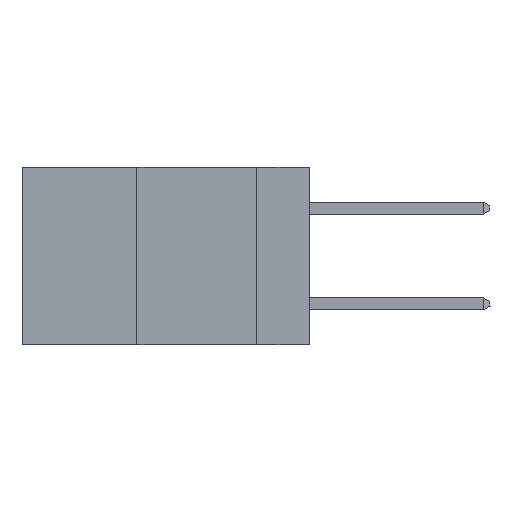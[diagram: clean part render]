
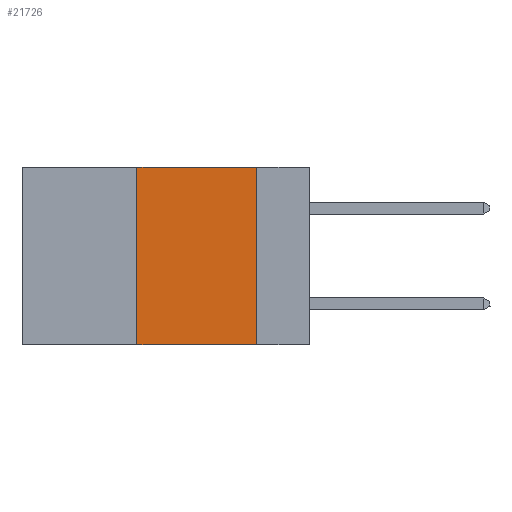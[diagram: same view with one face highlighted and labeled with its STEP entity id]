
A CAD part, left-side view. The second image highlights one B-rep face of the part: STEP entity #21726.
In plain terms, the highlighted planar face has unit normal (-1, 0, 0).
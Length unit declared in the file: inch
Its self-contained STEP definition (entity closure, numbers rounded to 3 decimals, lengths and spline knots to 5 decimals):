
#480 = DIRECTION ( 'NONE',  ( 0., -1., 0. ) ) ;
#1325 = LINE ( 'NONE', #21217, #25926 ) ;
#3565 = VERTEX_POINT ( 'NONE', #12409 ) ;
#3645 = DIRECTION ( 'NONE',  ( 0., 0., -1. ) ) ;
#3710 = CARTESIAN_POINT ( 'NONE',  ( 0., 0.36, 0. ) ) ;
#4708 = ORIENTED_EDGE ( 'NONE', *, *, #20741, .F. ) ;
#4758 = FACE_OUTER_BOUND ( 'NONE', #24506, .T. ) ;
#5833 = EDGE_CURVE ( 'NONE', #11172, #9596, #7751, .T. ) ;
#6070 = ORIENTED_EDGE ( 'NONE', *, *, #13353, .F. ) ;
#7751 = LINE ( 'NONE', #9985, #20923 ) ;
#7928 = DIRECTION ( 'NONE',  ( 0., 0., 1. ) ) ;
#8585 = DIRECTION ( 'NONE',  ( 1., 0., 0. ) ) ;
#9596 = VERTEX_POINT ( 'NONE', #22916 ) ;
#9985 = CARTESIAN_POINT ( 'NONE',  ( 0., 0.6, -0.37 ) ) ;
#11172 = VERTEX_POINT ( 'NONE', #24205 ) ;
#12095 = DIRECTION ( 'NONE',  ( 0., -1., 0. ) ) ;
#12096 = ORIENTED_EDGE ( 'NONE', *, *, #5833, .T. ) ;
#12409 = CARTESIAN_POINT ( 'NONE',  ( 0., 0.36, 0. ) ) ;
#12434 = LINE ( 'NONE', #26424, #12753 ) ;
#12753 = VECTOR ( 'NONE', #3645, 39.37008 ) ;
#13096 = EDGE_CURVE ( 'NONE', #26324, #9596, #12434, .T. ) ;
#13353 = EDGE_CURVE ( 'NONE', #3565, #26324, #1325, .T. ) ;
#13358 = ORIENTED_EDGE ( 'NONE', *, *, #13096, .F. ) ;
#13376 = CARTESIAN_POINT ( 'NONE',  ( 0., 0.11, 0. ) ) ;
#16861 = LINE ( 'NONE', #3710, #17170 ) ;
#17170 = VECTOR ( 'NONE', #7928, 39.37008 ) ;
#19977 = AXIS2_PLACEMENT_3D ( 'NONE', #23495, #8585, #23300 ) ;
#20741 = EDGE_CURVE ( 'NONE', #11172, #3565, #16861, .T. ) ;
#20923 = VECTOR ( 'NONE', #12095, 39.37008 ) ;
#21214 = PLANE ( 'NONE',  #19977 ) ;
#21217 = CARTESIAN_POINT ( 'NONE',  ( 0., 0.6, 0. ) ) ;
#21726 = ADVANCED_FACE ( 'NONE', ( #4758 ), #21214, .F. ) ;
#22916 = CARTESIAN_POINT ( 'NONE',  ( 0., 0.11, -0.37 ) ) ;
#23300 = DIRECTION ( 'NONE',  ( 0., 0., -1. ) ) ;
#23495 = CARTESIAN_POINT ( 'NONE',  ( 0., 0.6, 0. ) ) ;
#24205 = CARTESIAN_POINT ( 'NONE',  ( 0., 0.36, -0.37 ) ) ;
#24506 = EDGE_LOOP ( 'NONE', ( #13358, #6070, #4708, #12096 ) ) ;
#25926 = VECTOR ( 'NONE', #480, 39.37008 ) ;
#26324 = VERTEX_POINT ( 'NONE', #13376 ) ;
#26424 = CARTESIAN_POINT ( 'NONE',  ( 0., 0.11, 0. ) ) ;
